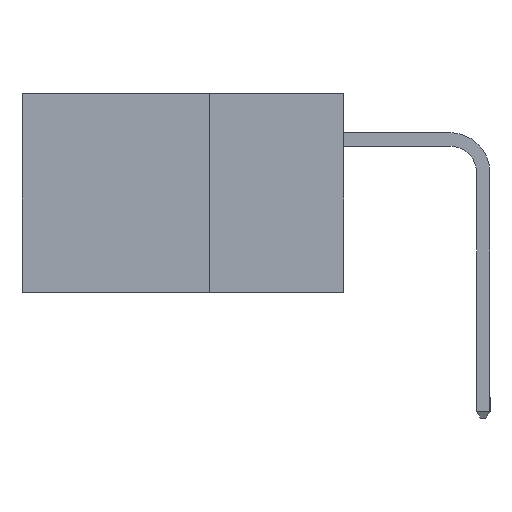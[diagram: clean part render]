
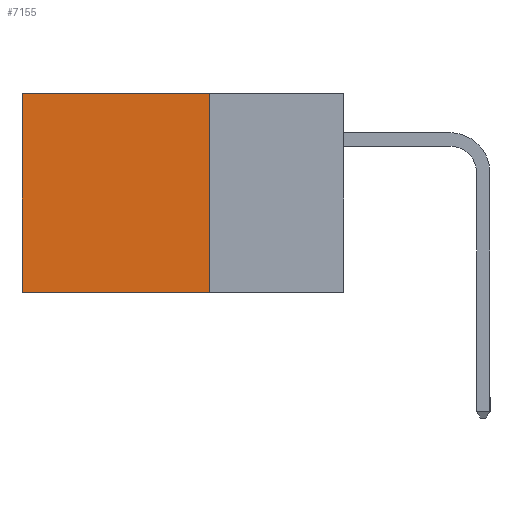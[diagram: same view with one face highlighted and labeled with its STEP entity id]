
A CAD part, left-side view. The second image highlights one B-rep face of the part: STEP entity #7155.
In plain terms, the highlighted planar face has unit normal (-1, 0, 0).
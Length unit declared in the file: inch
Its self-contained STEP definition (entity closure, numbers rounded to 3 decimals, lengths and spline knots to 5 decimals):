
#2016 = EDGE_LOOP ( 'NONE', ( #20635, #13109, #19511, #16824 ) ) ;
#2181 = DIRECTION ( 'NONE',  ( 0., 0., -1. ) ) ;
#2204 = LINE ( 'NONE', #20252, #14785 ) ;
#3238 = DIRECTION ( 'NONE',  ( 0., 1., 0. ) ) ;
#3736 = VECTOR ( 'NONE', #3238, 39.37008 ) ;
#6003 = DIRECTION ( 'NONE',  ( 0., 0., -1. ) ) ;
#6069 = DIRECTION ( 'NONE',  ( 1., 0., 0. ) ) ;
#6148 = VECTOR ( 'NONE', #12019, 39.37008 ) ;
#6239 = CARTESIAN_POINT ( 'NONE',  ( 0.2615, 0.6, 0. ) ) ;
#6914 = VERTEX_POINT ( 'NONE', #7280 ) ;
#7155 = ADVANCED_FACE ( 'NONE', ( #15326 ), #11934, .F. ) ;
#7280 = CARTESIAN_POINT ( 'NONE',  ( 0.2615, 0.25, 0. ) ) ;
#7632 = VERTEX_POINT ( 'NONE', #17013 ) ;
#8317 = DIRECTION ( 'NONE',  ( 0., 0., -1. ) ) ;
#8428 = CARTESIAN_POINT ( 'NONE',  ( 0.2615, 0.25, -0.37 ) ) ;
#9611 = VERTEX_POINT ( 'NONE', #6239 ) ;
#10765 = CARTESIAN_POINT ( 'NONE',  ( 0.2615, 0.6, -0.37 ) ) ;
#11715 = LINE ( 'NONE', #10765, #15673 ) ;
#11934 = PLANE ( 'NONE',  #18777 ) ;
#12019 = DIRECTION ( 'NONE',  ( 0., 1., 0. ) ) ;
#12064 = CARTESIAN_POINT ( 'NONE',  ( 0.2615, 0.25, -0.37 ) ) ;
#13109 = ORIENTED_EDGE ( 'NONE', *, *, #17089, .F. ) ;
#13601 = EDGE_CURVE ( 'NONE', #6914, #9611, #15773, .T. ) ;
#14785 = VECTOR ( 'NONE', #8317, 39.37008 ) ;
#14934 = VERTEX_POINT ( 'NONE', #15510 ) ;
#15326 = FACE_OUTER_BOUND ( 'NONE', #2016, .T. ) ;
#15408 = CARTESIAN_POINT ( 'NONE',  ( 0.2615, 0.25, 0. ) ) ;
#15494 = EDGE_CURVE ( 'NONE', #6914, #7632, #2204, .T. ) ;
#15510 = CARTESIAN_POINT ( 'NONE',  ( 0.2615, 0.6, -0.37 ) ) ;
#15673 = VECTOR ( 'NONE', #2181, 39.37008 ) ;
#15773 = LINE ( 'NONE', #15408, #6148 ) ;
#16824 = ORIENTED_EDGE ( 'NONE', *, *, #13601, .T. ) ;
#16825 = LINE ( 'NONE', #8428, #3736 ) ;
#17013 = CARTESIAN_POINT ( 'NONE',  ( 0.2615, 0.25, -0.37 ) ) ;
#17089 = EDGE_CURVE ( 'NONE', #7632, #14934, #16825, .T. ) ;
#18777 = AXIS2_PLACEMENT_3D ( 'NONE', #12064, #6069, #6003 ) ;
#19511 = ORIENTED_EDGE ( 'NONE', *, *, #15494, .F. ) ;
#20252 = CARTESIAN_POINT ( 'NONE',  ( 0.2615, 0.25, -0.37 ) ) ;
#20635 = ORIENTED_EDGE ( 'NONE', *, *, #21916, .T. ) ;
#21916 = EDGE_CURVE ( 'NONE', #9611, #14934, #11715, .T. ) ;
